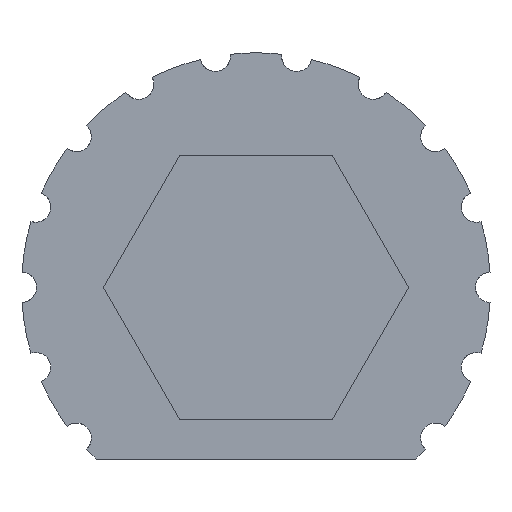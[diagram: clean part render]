
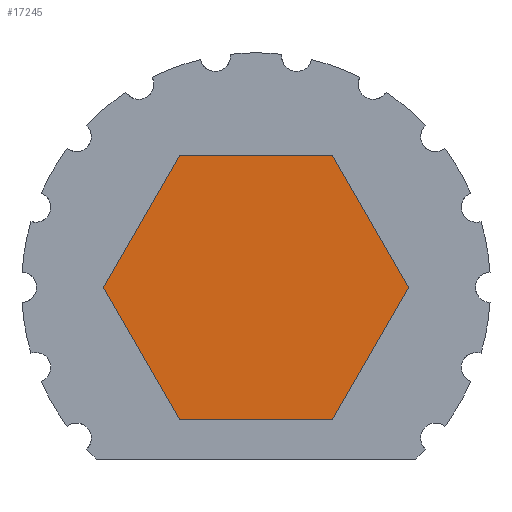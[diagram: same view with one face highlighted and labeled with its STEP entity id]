
A CAD part, left-side view. The second image highlights one B-rep face of the part: STEP entity #17245.
In plain terms, the highlighted planar face has unit normal (-1, 0, 0).
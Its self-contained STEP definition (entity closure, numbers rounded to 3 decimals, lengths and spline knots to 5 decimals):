
#974 = CARTESIAN_POINT ( 'NONE',  ( -0.2, 0.16445, 0. ) ) ;
#1160 = VECTOR ( 'NONE', #25745, 39.37008 ) ;
#1725 = VECTOR ( 'NONE', #11111, 39.37008 ) ;
#1829 = LINE ( 'NONE', #2863, #1160 ) ;
#1946 = EDGE_CURVE ( 'NONE', #15542, #21217, #26806, .T. ) ;
#2144 = VECTOR ( 'NONE', #20043, 39.37008 ) ;
#2697 = CARTESIAN_POINT ( 'NONE',  ( -0.2, -0.08223, -0.14242 ) ) ;
#2863 = CARTESIAN_POINT ( 'NONE',  ( -0.2, 0.16445, 0. ) ) ;
#5989 = EDGE_CURVE ( 'NONE', #12656, #15542, #11526, .T. ) ;
#6643 = CARTESIAN_POINT ( 'NONE',  ( -0.2, -0.16445, 0. ) ) ;
#6668 = DIRECTION ( 'NONE',  ( 0., 0.5, 0.866 ) ) ;
#6744 = ORIENTED_EDGE ( 'NONE', *, *, #5989, .T. ) ;
#7210 = LINE ( 'NONE', #9406, #1725 ) ;
#7241 = CARTESIAN_POINT ( 'NONE',  ( -0.2, 0.08223, 0.14242 ) ) ;
#7620 = VECTOR ( 'NONE', #21275, 39.37008 ) ;
#9406 = CARTESIAN_POINT ( 'NONE',  ( -0.2, -0.08223, -0.14242 ) ) ;
#9412 = VERTEX_POINT ( 'NONE', #2697 ) ;
#9532 = CARTESIAN_POINT ( 'NONE',  ( -0.2, 0.08223, 0.14242 ) ) ;
#10071 = EDGE_CURVE ( 'NONE', #21217, #16458, #1829, .T. ) ;
#10312 = ORIENTED_EDGE ( 'NONE', *, *, #25013, .T. ) ;
#10353 = CARTESIAN_POINT ( 'NONE',  ( -0.2, 0., 0. ) ) ;
#10690 = DIRECTION ( 'NONE',  ( -1., 0., 0. ) ) ;
#11102 = VERTEX_POINT ( 'NONE', #6643 ) ;
#11111 = DIRECTION ( 'NONE',  ( 0., -0.5, 0.866 ) ) ;
#11526 = LINE ( 'NONE', #15887, #2144 ) ;
#12523 = VECTOR ( 'NONE', #23883, 39.37008 ) ;
#12589 = LINE ( 'NONE', #25284, #14217 ) ;
#12656 = VERTEX_POINT ( 'NONE', #13352 ) ;
#12750 = PLANE ( 'NONE',  #16062 ) ;
#13352 = CARTESIAN_POINT ( 'NONE',  ( -0.2, -0.08223, 0.14242 ) ) ;
#13681 = EDGE_CURVE ( 'NONE', #16458, #9412, #14675, .T. ) ;
#14217 = VECTOR ( 'NONE', #6668, 39.37008 ) ;
#14675 = LINE ( 'NONE', #17114, #7620 ) ;
#15508 = ORIENTED_EDGE ( 'NONE', *, *, #13681, .T. ) ;
#15542 = VERTEX_POINT ( 'NONE', #7241 ) ;
#15887 = CARTESIAN_POINT ( 'NONE',  ( -0.2, -0.08223, 0.14242 ) ) ;
#16062 = AXIS2_PLACEMENT_3D ( 'NONE', #10353, #10690, #22735 ) ;
#16458 = VERTEX_POINT ( 'NONE', #19039 ) ;
#17114 = CARTESIAN_POINT ( 'NONE',  ( -0.2, 0.08223, -0.14242 ) ) ;
#17245 = ADVANCED_FACE ( 'NONE', ( #19143 ), #12750, .T. ) ;
#18524 = ORIENTED_EDGE ( 'NONE', *, *, #1946, .T. ) ;
#18707 = EDGE_CURVE ( 'NONE', #9412, #11102, #7210, .T. ) ;
#19039 = CARTESIAN_POINT ( 'NONE',  ( -0.2, 0.08223, -0.14242 ) ) ;
#19143 = FACE_OUTER_BOUND ( 'NONE', #22960, .T. ) ;
#20043 = DIRECTION ( 'NONE',  ( 0., 1., 0. ) ) ;
#20370 = ORIENTED_EDGE ( 'NONE', *, *, #18707, .T. ) ;
#21217 = VERTEX_POINT ( 'NONE', #974 ) ;
#21275 = DIRECTION ( 'NONE',  ( 0., -1., 0. ) ) ;
#22735 = DIRECTION ( 'NONE',  ( 0., 0., 1. ) ) ;
#22960 = EDGE_LOOP ( 'NONE', ( #20370, #10312, #6744, #18524, #25248, #15508 ) ) ;
#23883 = DIRECTION ( 'NONE',  ( 0., 0.5, -0.866 ) ) ;
#25013 = EDGE_CURVE ( 'NONE', #11102, #12656, #12589, .T. ) ;
#25248 = ORIENTED_EDGE ( 'NONE', *, *, #10071, .T. ) ;
#25284 = CARTESIAN_POINT ( 'NONE',  ( -0.2, -0.16445, 0. ) ) ;
#25745 = DIRECTION ( 'NONE',  ( 0., -0.5, -0.866 ) ) ;
#26806 = LINE ( 'NONE', #9532, #12523 ) ;
